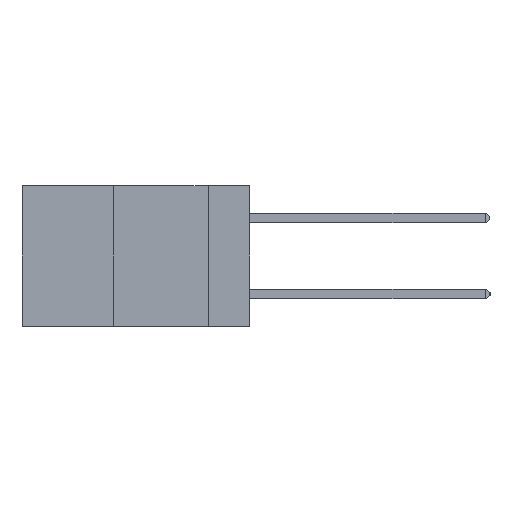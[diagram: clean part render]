
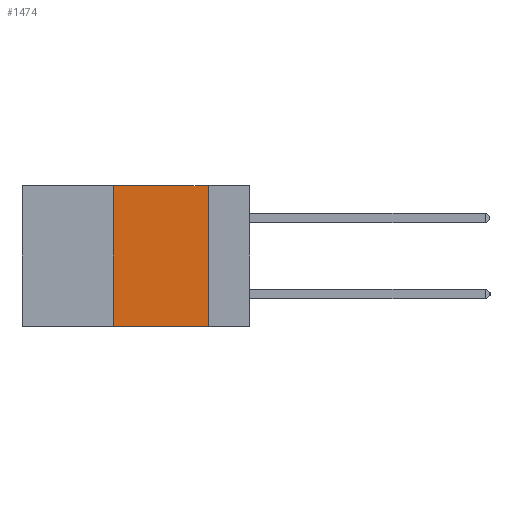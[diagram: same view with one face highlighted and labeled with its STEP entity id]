
A CAD part, left-side view. The second image highlights one B-rep face of the part: STEP entity #1474.
In plain terms, the highlighted planar face has unit normal (-1, 0, 0).
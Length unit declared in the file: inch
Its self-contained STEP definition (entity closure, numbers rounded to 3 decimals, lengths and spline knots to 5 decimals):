
#136 = EDGE_CURVE ( 'NONE', #7190, #10865, #11137, .T. ) ;
#414 = EDGE_CURVE ( 'NONE', #12045, #12364, #3287, .T. ) ;
#1100 = CARTESIAN_POINT ( 'NONE',  ( 0., 0.6, -0.37 ) ) ;
#1265 = CARTESIAN_POINT ( 'NONE',  ( 0., 0.11, 0. ) ) ;
#1430 = LINE ( 'NONE', #4952, #6376 ) ;
#1474 = ADVANCED_FACE ( 'NONE', ( #8831 ), #5946, .F. ) ;
#1534 = CARTESIAN_POINT ( 'NONE',  ( 0., 0.36, 0. ) ) ;
#1734 = CARTESIAN_POINT ( 'NONE',  ( 0., 0.11, 0. ) ) ;
#1895 = CARTESIAN_POINT ( 'NONE',  ( 0., 0.6, 0. ) ) ;
#2175 = DIRECTION ( 'NONE',  ( 0., -1., 0. ) ) ;
#3087 = VECTOR ( 'NONE', #6561, 39.37008 ) ;
#3197 = ORIENTED_EDGE ( 'NONE', *, *, #4872, .F. ) ;
#3287 = LINE ( 'NONE', #1895, #6569 ) ;
#3764 = LINE ( 'NONE', #1265, #3087 ) ;
#3903 = CARTESIAN_POINT ( 'NONE',  ( 0., 0.11, -0.37 ) ) ;
#4872 = EDGE_CURVE ( 'NONE', #12364, #10865, #3764, .T. ) ;
#4924 = ORIENTED_EDGE ( 'NONE', *, *, #414, .F. ) ;
#4952 = CARTESIAN_POINT ( 'NONE',  ( 0., 0.36, 0. ) ) ;
#5327 = EDGE_CURVE ( 'NONE', #7190, #12045, #1430, .T. ) ;
#5946 = PLANE ( 'NONE',  #10402 ) ;
#6223 = DIRECTION ( 'NONE',  ( 0., 0., 1. ) ) ;
#6376 = VECTOR ( 'NONE', #6223, 39.37008 ) ;
#6561 = DIRECTION ( 'NONE',  ( 0., 0., -1. ) ) ;
#6569 = VECTOR ( 'NONE', #8166, 39.37008 ) ;
#7190 = VERTEX_POINT ( 'NONE', #7860 ) ;
#7860 = CARTESIAN_POINT ( 'NONE',  ( 0., 0.36, -0.37 ) ) ;
#7874 = DIRECTION ( 'NONE',  ( 1., 0., 0. ) ) ;
#8166 = DIRECTION ( 'NONE',  ( 0., -1., 0. ) ) ;
#8693 = VECTOR ( 'NONE', #2175, 39.37008 ) ;
#8831 = FACE_OUTER_BOUND ( 'NONE', #10379, .T. ) ;
#9907 = CARTESIAN_POINT ( 'NONE',  ( 0., 0.6, 0. ) ) ;
#10379 = EDGE_LOOP ( 'NONE', ( #3197, #4924, #13412, #13287 ) ) ;
#10402 = AXIS2_PLACEMENT_3D ( 'NONE', #9907, #7874, #12102 ) ;
#10865 = VERTEX_POINT ( 'NONE', #3903 ) ;
#11137 = LINE ( 'NONE', #1100, #8693 ) ;
#12045 = VERTEX_POINT ( 'NONE', #1534 ) ;
#12102 = DIRECTION ( 'NONE',  ( 0., 0., -1. ) ) ;
#12364 = VERTEX_POINT ( 'NONE', #1734 ) ;
#13287 = ORIENTED_EDGE ( 'NONE', *, *, #136, .T. ) ;
#13412 = ORIENTED_EDGE ( 'NONE', *, *, #5327, .F. ) ;
